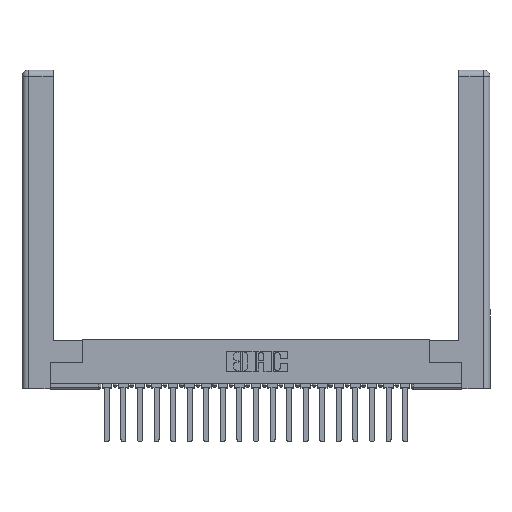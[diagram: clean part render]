
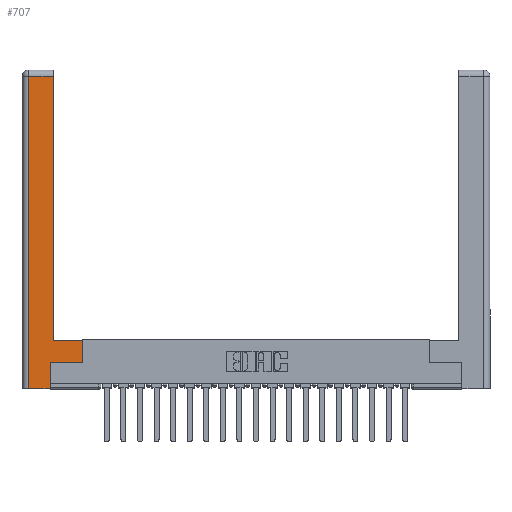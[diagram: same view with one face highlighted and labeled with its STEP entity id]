
A CAD part, top view. The second image highlights one B-rep face of the part: STEP entity #707.
In plain terms, the highlighted planar face has unit normal (0, 0, 1).
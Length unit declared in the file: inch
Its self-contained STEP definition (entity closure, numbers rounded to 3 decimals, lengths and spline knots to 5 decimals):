
#171 = CARTESIAN_POINT ( 'NONE',  ( 0.265, 0., 0. ) ) ;
#707 = ADVANCED_FACE ( 'NONE', ( #3158 ), #19503, .F. ) ;
#899 = LINE ( 'NONE', #16447, #21525 ) ;
#1100 = DIRECTION ( 'NONE',  ( 1., 0., 0. ) ) ;
#1802 = ORIENTED_EDGE ( 'NONE', *, *, #19125, .T. ) ;
#1888 = DIRECTION ( 'NONE',  ( 0., 1., 0. ) ) ;
#1913 = CARTESIAN_POINT ( 'NONE',  ( 0.0615, 0., 0. ) ) ;
#1987 = DIRECTION ( 'NONE',  ( 0., -1., 0. ) ) ;
#2019 = VERTEX_POINT ( 'NONE', #18619 ) ;
#2426 = DIRECTION ( 'NONE',  ( -1., 0., 0. ) ) ;
#2465 = ORIENTED_EDGE ( 'NONE', *, *, #22097, .T. ) ;
#2485 = DIRECTION ( 'NONE',  ( -1., 0., 0. ) ) ;
#3158 = FACE_OUTER_BOUND ( 'NONE', #21356, .T. ) ;
#3877 = VERTEX_POINT ( 'NONE', #17606 ) ;
#4046 = VECTOR ( 'NONE', #1987, 39.37008 ) ;
#4132 = ORIENTED_EDGE ( 'NONE', *, *, #5097, .T. ) ;
#5016 = DIRECTION ( 'NONE',  ( 0., 1., 0. ) ) ;
#5097 = EDGE_CURVE ( 'NONE', #5553, #21480, #13319, .T. ) ;
#5425 = CARTESIAN_POINT ( 'NONE',  ( 0.0615, 0., 0. ) ) ;
#5553 = VERTEX_POINT ( 'NONE', #9296 ) ;
#5564 = EDGE_CURVE ( 'NONE', #13258, #3877, #7613, .T. ) ;
#5782 = ORIENTED_EDGE ( 'NONE', *, *, #20023, .T. ) ;
#6145 = DIRECTION ( 'NONE',  ( -1., 0., 0. ) ) ;
#6280 = VECTOR ( 'NONE', #6145, 39.37008 ) ;
#7613 = LINE ( 'NONE', #16093, #6280 ) ;
#8935 = CARTESIAN_POINT ( 'NONE',  ( 0.295, 2.94, 0. ) ) ;
#9114 = CARTESIAN_POINT ( 'NONE',  ( 0., 0., 0. ) ) ;
#9296 = CARTESIAN_POINT ( 'NONE',  ( 0.565, 0.45, 0. ) ) ;
#9320 = VECTOR ( 'NONE', #1888, 39.37008 ) ;
#9654 = ORIENTED_EDGE ( 'NONE', *, *, #18003, .T. ) ;
#9923 = LINE ( 'NONE', #20074, #15307 ) ;
#10605 = VECTOR ( 'NONE', #2485, 39.37008 ) ;
#10996 = DIRECTION ( 'NONE',  ( 0., 0., -1. ) ) ;
#11343 = EDGE_CURVE ( 'NONE', #21480, #13258, #12886, .T. ) ;
#11441 = LINE ( 'NONE', #22465, #12505 ) ;
#11795 = ORIENTED_EDGE ( 'NONE', *, *, #12527, .T. ) ;
#12223 = ORIENTED_EDGE ( 'NONE', *, *, #5564, .T. ) ;
#12505 = VECTOR ( 'NONE', #5016, 39.37008 ) ;
#12527 = EDGE_CURVE ( 'NONE', #13178, #21656, #13914, .T. ) ;
#12886 = LINE ( 'NONE', #19402, #16690 ) ;
#13178 = VERTEX_POINT ( 'NONE', #171 ) ;
#13258 = VERTEX_POINT ( 'NONE', #8935 ) ;
#13319 = LINE ( 'NONE', #16420, #10605 ) ;
#13914 = LINE ( 'NONE', #17410, #9320 ) ;
#15307 = VECTOR ( 'NONE', #1100, 39.37008 ) ;
#15418 = ORIENTED_EDGE ( 'NONE', *, *, #11343, .T. ) ;
#15643 = LINE ( 'NONE', #5425, #4046 ) ;
#16093 = CARTESIAN_POINT ( 'NONE',  ( 0.0615, 2.94, 0. ) ) ;
#16420 = CARTESIAN_POINT ( 'NONE',  ( 0.295, 0.45, 0. ) ) ;
#16447 = CARTESIAN_POINT ( 'NONE',  ( 0.265, 0., 0. ) ) ;
#16574 = VERTEX_POINT ( 'NONE', #1913 ) ;
#16690 = VECTOR ( 'NONE', #19333, 39.37008 ) ;
#17410 = CARTESIAN_POINT ( 'NONE',  ( 0.265, 0.245, 0. ) ) ;
#17519 = AXIS2_PLACEMENT_3D ( 'NONE', #9114, #10996, #2426 ) ;
#17606 = CARTESIAN_POINT ( 'NONE',  ( 0.0615, 2.94, 0. ) ) ;
#17916 = CARTESIAN_POINT ( 'NONE',  ( 0.295, 0.45, 0. ) ) ;
#18003 = EDGE_CURVE ( 'NONE', #21656, #2019, #9923, .T. ) ;
#18619 = CARTESIAN_POINT ( 'NONE',  ( 0.565, 0.245, 0. ) ) ;
#19125 = EDGE_CURVE ( 'NONE', #16574, #13178, #899, .T. ) ;
#19333 = DIRECTION ( 'NONE',  ( 0., 1., 0. ) ) ;
#19402 = CARTESIAN_POINT ( 'NONE',  ( 0.295, 3., 0. ) ) ;
#19503 = PLANE ( 'NONE',  #17519 ) ;
#20023 = EDGE_CURVE ( 'NONE', #2019, #5553, #11441, .T. ) ;
#20074 = CARTESIAN_POINT ( 'NONE',  ( 0.565, 0.245, 0. ) ) ;
#21356 = EDGE_LOOP ( 'NONE', ( #15418, #12223, #2465, #1802, #11795, #9654, #5782, #4132 ) ) ;
#21480 = VERTEX_POINT ( 'NONE', #17916 ) ;
#21525 = VECTOR ( 'NONE', #21698, 39.37008 ) ;
#21637 = CARTESIAN_POINT ( 'NONE',  ( 0.265, 0.245, 0. ) ) ;
#21656 = VERTEX_POINT ( 'NONE', #21637 ) ;
#21698 = DIRECTION ( 'NONE',  ( 1., 0., 0. ) ) ;
#22097 = EDGE_CURVE ( 'NONE', #3877, #16574, #15643, .T. ) ;
#22465 = CARTESIAN_POINT ( 'NONE',  ( 0.565, 0.45, 0. ) ) ;
